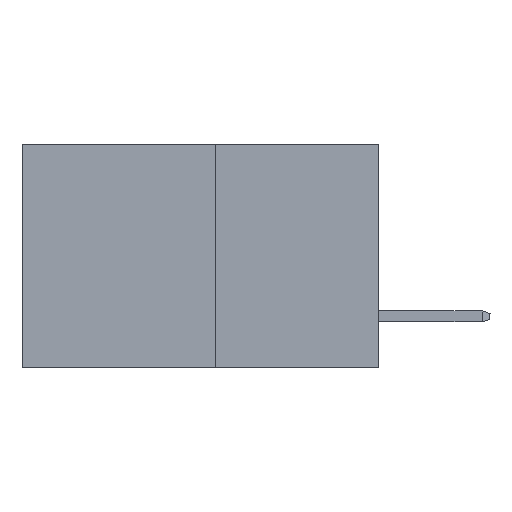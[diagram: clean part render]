
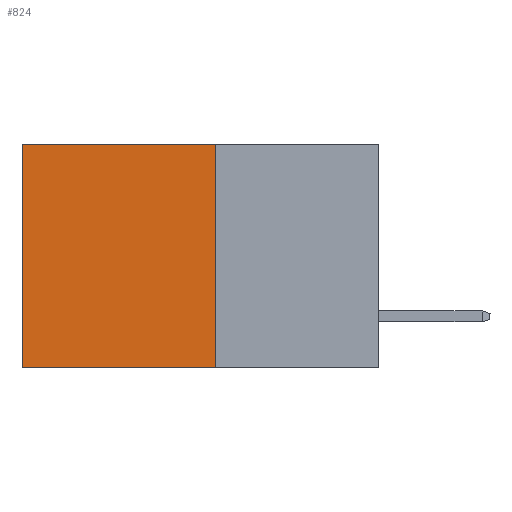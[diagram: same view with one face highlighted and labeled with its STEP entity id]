
A CAD part, left-side view. The second image highlights one B-rep face of the part: STEP entity #824.
In plain terms, the highlighted planar face has unit normal (-1, 0, 0).
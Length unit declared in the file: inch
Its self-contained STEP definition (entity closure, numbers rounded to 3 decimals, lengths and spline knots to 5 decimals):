
#130 = CARTESIAN_POINT ( 'NONE',  ( 0.277, 0.59, 0. ) ) ;
#440 = CARTESIAN_POINT ( 'NONE',  ( 0.277, 0.59, -0.37 ) ) ;
#569 = VERTEX_POINT ( 'NONE', #8935 ) ;
#824 = ADVANCED_FACE ( 'NONE', ( #7344 ), #5095, .F. ) ;
#1038 = EDGE_CURVE ( 'NONE', #1869, #2342, #8558, .T. ) ;
#1255 = AXIS2_PLACEMENT_3D ( 'NONE', #4460, #4769, #5120 ) ;
#1279 = VECTOR ( 'NONE', #1358, 39.37008 ) ;
#1293 = ORIENTED_EDGE ( 'NONE', *, *, #4268, .T. ) ;
#1358 = DIRECTION ( 'NONE',  ( 0., 0., -1. ) ) ;
#1379 = VECTOR ( 'NONE', #1857, 39.37008 ) ;
#1541 = VECTOR ( 'NONE', #5122, 39.37008 ) ;
#1850 = EDGE_CURVE ( 'NONE', #7482, #2342, #7685, .T. ) ;
#1857 = DIRECTION ( 'NONE',  ( 0., 0., -1. ) ) ;
#1869 = VERTEX_POINT ( 'NONE', #2329 ) ;
#2329 = CARTESIAN_POINT ( 'NONE',  ( 0.277, 0.27, -0.37 ) ) ;
#2342 = VERTEX_POINT ( 'NONE', #440 ) ;
#2923 = EDGE_CURVE ( 'NONE', #569, #1869, #3646, .T. ) ;
#3024 = ORIENTED_EDGE ( 'NONE', *, *, #2923, .F. ) ;
#3129 = EDGE_LOOP ( 'NONE', ( #9653, #8885, #3024, #1293 ) ) ;
#3646 = LINE ( 'NONE', #3997, #1379 ) ;
#3997 = CARTESIAN_POINT ( 'NONE',  ( 0.277, 0.27, -0.37 ) ) ;
#4233 = CARTESIAN_POINT ( 'NONE',  ( 0.277, 0.59, -0.37 ) ) ;
#4268 = EDGE_CURVE ( 'NONE', #569, #7482, #7913, .T. ) ;
#4460 = CARTESIAN_POINT ( 'NONE',  ( 0.277, 0.27, -0.37 ) ) ;
#4611 = VECTOR ( 'NONE', #8435, 39.37008 ) ;
#4769 = DIRECTION ( 'NONE',  ( 1., 0., 0. ) ) ;
#5095 = PLANE ( 'NONE',  #1255 ) ;
#5120 = DIRECTION ( 'NONE',  ( 0., 0., -1. ) ) ;
#5122 = DIRECTION ( 'NONE',  ( 0., 1., 0. ) ) ;
#7344 = FACE_OUTER_BOUND ( 'NONE', #3129, .T. ) ;
#7482 = VERTEX_POINT ( 'NONE', #130 ) ;
#7685 = LINE ( 'NONE', #4233, #1279 ) ;
#7913 = LINE ( 'NONE', #9835, #1541 ) ;
#8435 = DIRECTION ( 'NONE',  ( 0., 1., 0. ) ) ;
#8558 = LINE ( 'NONE', #9233, #4611 ) ;
#8885 = ORIENTED_EDGE ( 'NONE', *, *, #1038, .F. ) ;
#8935 = CARTESIAN_POINT ( 'NONE',  ( 0.277, 0.27, 0. ) ) ;
#9233 = CARTESIAN_POINT ( 'NONE',  ( 0.277, 0.27, -0.37 ) ) ;
#9653 = ORIENTED_EDGE ( 'NONE', *, *, #1850, .T. ) ;
#9835 = CARTESIAN_POINT ( 'NONE',  ( 0.277, 0.27, 0. ) ) ;
